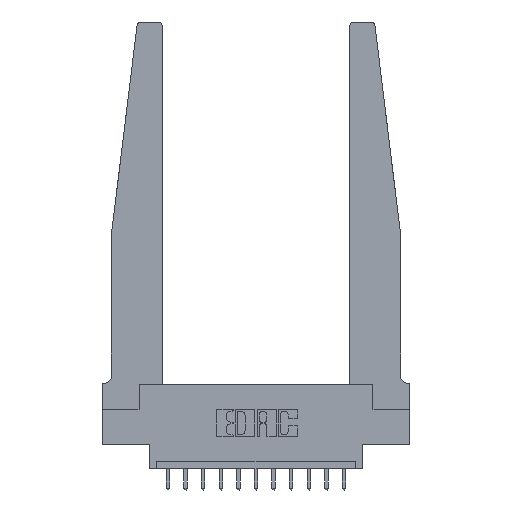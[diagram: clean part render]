
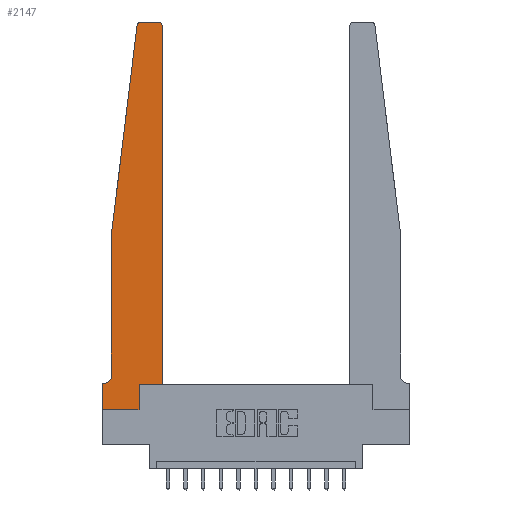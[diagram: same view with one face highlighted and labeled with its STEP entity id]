
A CAD part, top view. The second image highlights one B-rep face of the part: STEP entity #2147.
In plain terms, the highlighted planar face has unit normal (0, 0, 1).
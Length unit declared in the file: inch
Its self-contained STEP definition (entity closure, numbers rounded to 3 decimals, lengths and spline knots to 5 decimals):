
#134 = CARTESIAN_POINT ( 'NONE',  ( 0.24675, 2.72367, 0.37 ) ) ;
#285 = ORIENTED_EDGE ( 'NONE', *, *, #11619, .T. ) ;
#324 = VECTOR ( 'NONE', #11270, 39.37008 ) ;
#371 = DIRECTION ( 'NONE',  ( 0., 0., -1. ) ) ;
#443 = ORIENTED_EDGE ( 'NONE', *, *, #14473, .T. ) ;
#554 = CARTESIAN_POINT ( 'NONE',  ( 0.2605, 0.18, 0.37 ) ) ;
#1117 = AXIS2_PLACEMENT_3D ( 'NONE', #6187, #3457, #12603 ) ;
#1349 = VERTEX_POINT ( 'NONE', #9116 ) ;
#1761 = AXIS2_PLACEMENT_3D ( 'NONE', #6941, #7107, #4544 ) ;
#1891 = DIRECTION ( 'NONE',  ( 1., 0., 0. ) ) ;
#2147 = ADVANCED_FACE ( 'NONE', ( #5718 ), #4493, .T. ) ;
#2731 = VERTEX_POINT ( 'NONE', #13450 ) ;
#2788 = LINE ( 'NONE', #12013, #8938 ) ;
#3457 = DIRECTION ( 'NONE',  ( 0., 0., 1. ) ) ;
#3597 = ORIENTED_EDGE ( 'NONE', *, *, #6075, .T. ) ;
#3637 = VECTOR ( 'NONE', #9667, 39.37008 ) ;
#3822 = VERTEX_POINT ( 'NONE', #10048 ) ;
#4066 = CARTESIAN_POINT ( 'NONE',  ( 0.015, 0.1875, 0.37 ) ) ;
#4067 = EDGE_CURVE ( 'NONE', #2731, #5203, #16316, .T. ) ;
#4333 = ORIENTED_EDGE ( 'NONE', *, *, #9501, .T. ) ;
#4493 = PLANE ( 'NONE',  #13972 ) ;
#4544 = DIRECTION ( 'NONE',  ( 1., 0., 0. ) ) ;
#4790 = CARTESIAN_POINT ( 'NONE',  ( 0.065, 1.25, 0.37 ) ) ;
#5184 = VERTEX_POINT ( 'NONE', #134 ) ;
#5203 = VERTEX_POINT ( 'NONE', #4066 ) ;
#5303 = LINE ( 'NONE', #554, #11462 ) ;
#5335 = LINE ( 'NONE', #15492, #14792 ) ;
#5584 = LINE ( 'NONE', #10589, #3637 ) ;
#5718 = FACE_OUTER_BOUND ( 'NONE', #14677, .T. ) ;
#5832 = EDGE_CURVE ( 'NONE', #15858, #3822, #6242, .T. ) ;
#6075 = EDGE_CURVE ( 'NONE', #10659, #12690, #15888, .T. ) ;
#6107 = ORIENTED_EDGE ( 'NONE', *, *, #14037, .T. ) ;
#6187 = CARTESIAN_POINT ( 'NONE',  ( 0.27653, 2.72, 0.37 ) ) ;
#6205 = EDGE_CURVE ( 'NONE', #12690, #8239, #14654, .T. ) ;
#6242 = CIRCLE ( 'NONE', #1761, 0.03 ) ;
#6532 = ORIENTED_EDGE ( 'NONE', *, *, #11526, .T. ) ;
#6926 = DIRECTION ( 'NONE',  ( -0.122, -0.992, 0. ) ) ;
#6941 = CARTESIAN_POINT ( 'NONE',  ( 0.395, 2.72, 0.37 ) ) ;
#7107 = DIRECTION ( 'NONE',  ( 0., 0., 1. ) ) ;
#7118 = VERTEX_POINT ( 'NONE', #10443 ) ;
#7490 = EDGE_CURVE ( 'NONE', #7118, #15858, #5584, .T. ) ;
#7841 = DIRECTION ( 'NONE',  ( -1., 0., 0. ) ) ;
#7933 = VECTOR ( 'NONE', #1891, 39.37008 ) ;
#8239 = VERTEX_POINT ( 'NONE', #9937 ) ;
#8254 = CARTESIAN_POINT ( 'NONE',  ( 0., 0., 0.37 ) ) ;
#8259 = EDGE_CURVE ( 'NONE', #3822, #1349, #5335, .T. ) ;
#8380 = EDGE_CURVE ( 'NONE', #5184, #10512, #2788, .T. ) ;
#8501 = LINE ( 'NONE', #10933, #7933 ) ;
#8938 = VECTOR ( 'NONE', #6926, 39.37008 ) ;
#9116 = CARTESIAN_POINT ( 'NONE',  ( 0.27653, 2.75, 0.37 ) ) ;
#9162 = AXIS2_PLACEMENT_3D ( 'NONE', #14046, #371, #11466 ) ;
#9252 = CARTESIAN_POINT ( 'NONE',  ( 0.2605, 0.18, 0.37 ) ) ;
#9501 = EDGE_CURVE ( 'NONE', #15696, #7118, #8501, .T. ) ;
#9503 = CARTESIAN_POINT ( 'NONE',  ( 0., 0., 0.37 ) ) ;
#9667 = DIRECTION ( 'NONE',  ( 0., 1., 0. ) ) ;
#9759 = ORIENTED_EDGE ( 'NONE', *, *, #7490, .T. ) ;
#9783 = CARTESIAN_POINT ( 'NONE',  ( 0.065, 0.1875, 0.37 ) ) ;
#9864 = ORIENTED_EDGE ( 'NONE', *, *, #6205, .T. ) ;
#9937 = CARTESIAN_POINT ( 'NONE',  ( 0.2605, 0., 0.37 ) ) ;
#10048 = CARTESIAN_POINT ( 'NONE',  ( 0.395, 2.75, 0.37 ) ) ;
#10443 = CARTESIAN_POINT ( 'NONE',  ( 0.425, 0.18, 0.37 ) ) ;
#10512 = VERTEX_POINT ( 'NONE', #10751 ) ;
#10589 = CARTESIAN_POINT ( 'NONE',  ( 0.425, 0.18, 0.37 ) ) ;
#10659 = VERTEX_POINT ( 'NONE', #13405 ) ;
#10751 = CARTESIAN_POINT ( 'NONE',  ( 0.065, 1.25, 0.37 ) ) ;
#10933 = CARTESIAN_POINT ( 'NONE',  ( 0.425, 0.18, 0.37 ) ) ;
#10988 = ORIENTED_EDGE ( 'NONE', *, *, #5832, .T. ) ;
#11067 = CARTESIAN_POINT ( 'NONE',  ( 0., 0.1875, 0.37 ) ) ;
#11270 = DIRECTION ( 'NONE',  ( 0., -1., 0. ) ) ;
#11445 = CIRCLE ( 'NONE', #1117, 0.03 ) ;
#11462 = VECTOR ( 'NONE', #11718, 39.37008 ) ;
#11466 = DIRECTION ( 'NONE',  ( -1., 0., 0. ) ) ;
#11526 = EDGE_CURVE ( 'NONE', #10512, #2731, #14753, .T. ) ;
#11619 = EDGE_CURVE ( 'NONE', #1349, #5184, #11445, .T. ) ;
#11718 = DIRECTION ( 'NONE',  ( 0., 1., 0. ) ) ;
#11841 = ORIENTED_EDGE ( 'NONE', *, *, #8380, .T. ) ;
#11926 = DIRECTION ( 'NONE',  ( 0., -1., 0. ) ) ;
#12013 = CARTESIAN_POINT ( 'NONE',  ( 0.065, 1.25, 0.37 ) ) ;
#12149 = ORIENTED_EDGE ( 'NONE', *, *, #4067, .T. ) ;
#12220 = DIRECTION ( 'NONE',  ( -1., 0., 0. ) ) ;
#12541 = LINE ( 'NONE', #9783, #15156 ) ;
#12603 = DIRECTION ( 'NONE',  ( 1., 0., 0. ) ) ;
#12632 = VECTOR ( 'NONE', #11926, 39.37008 ) ;
#12690 = VERTEX_POINT ( 'NONE', #15612 ) ;
#12995 = ORIENTED_EDGE ( 'NONE', *, *, #8259, .T. ) ;
#13245 = CARTESIAN_POINT ( 'NONE',  ( 0.425, 2.72, 0.37 ) ) ;
#13405 = CARTESIAN_POINT ( 'NONE',  ( 0., 0.1875, 0.37 ) ) ;
#13450 = CARTESIAN_POINT ( 'NONE',  ( 0.065, 0.2375, 0.37 ) ) ;
#13972 = AXIS2_PLACEMENT_3D ( 'NONE', #11067, #15032, #16101 ) ;
#14037 = EDGE_CURVE ( 'NONE', #5203, #10659, #12541, .T. ) ;
#14046 = CARTESIAN_POINT ( 'NONE',  ( 0.015, 0.2375, 0.37 ) ) ;
#14473 = EDGE_CURVE ( 'NONE', #8239, #15696, #5303, .T. ) ;
#14575 = DIRECTION ( 'NONE',  ( 1., 0., 0. ) ) ;
#14654 = LINE ( 'NONE', #9503, #16336 ) ;
#14677 = EDGE_LOOP ( 'NONE', ( #12995, #285, #11841, #6532, #12149, #6107, #3597, #9864, #443, #4333, #9759, #10988 ) ) ;
#14753 = LINE ( 'NONE', #4790, #324 ) ;
#14792 = VECTOR ( 'NONE', #7841, 39.37008 ) ;
#15032 = DIRECTION ( 'NONE',  ( 0., 0., 1. ) ) ;
#15156 = VECTOR ( 'NONE', #12220, 39.37008 ) ;
#15492 = CARTESIAN_POINT ( 'NONE',  ( 0.25, 2.75, 0.37 ) ) ;
#15612 = CARTESIAN_POINT ( 'NONE',  ( 0., 0., 0.37 ) ) ;
#15696 = VERTEX_POINT ( 'NONE', #9252 ) ;
#15858 = VERTEX_POINT ( 'NONE', #13245 ) ;
#15888 = LINE ( 'NONE', #8254, #12632 ) ;
#16101 = DIRECTION ( 'NONE',  ( 1., 0., 0. ) ) ;
#16316 = CIRCLE ( 'NONE', #9162, 0.05 ) ;
#16336 = VECTOR ( 'NONE', #14575, 39.37008 ) ;
